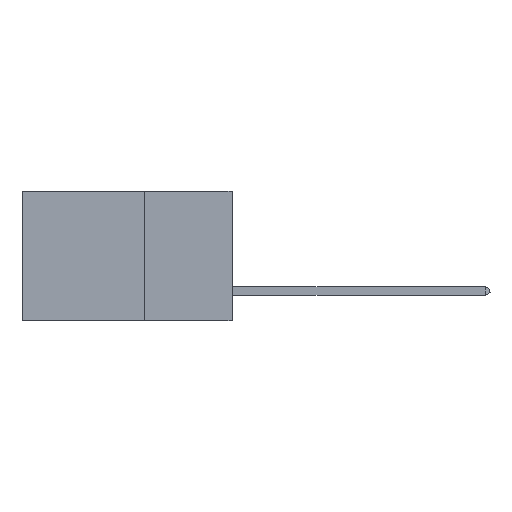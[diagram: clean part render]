
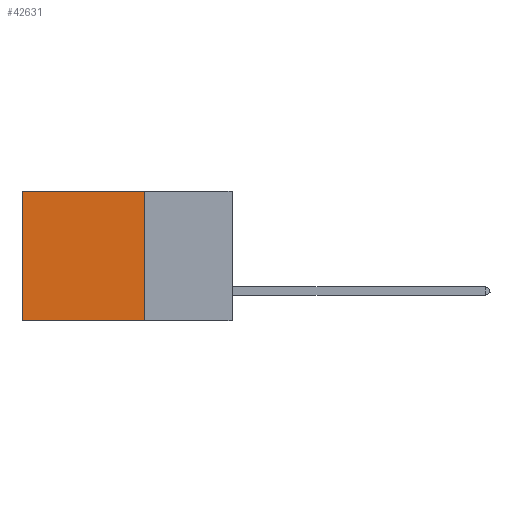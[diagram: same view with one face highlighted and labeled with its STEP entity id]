
A CAD part, left-side view. The second image highlights one B-rep face of the part: STEP entity #42631.
In plain terms, the highlighted planar face has unit normal (-1, 0, 0).
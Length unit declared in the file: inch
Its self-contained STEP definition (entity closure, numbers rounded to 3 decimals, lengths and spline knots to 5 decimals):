
#257 = EDGE_CURVE ( 'NONE', #31755, #35218, #38002, .T. ) ;
#869 = ORIENTED_EDGE ( 'NONE', *, *, #32308, .T. ) ;
#3611 = PLANE ( 'NONE',  #15359 ) ;
#4329 = DIRECTION ( 'NONE',  ( 0., 0., -1. ) ) ;
#5805 = EDGE_CURVE ( 'NONE', #31755, #28774, #27820, .T. ) ;
#6873 = VECTOR ( 'NONE', #4329, 39.37008 ) ;
#7428 = VECTOR ( 'NONE', #9564, 39.37008 ) ;
#7814 = CARTESIAN_POINT ( 'NONE',  ( 0.2875, 0.25, 0. ) ) ;
#9564 = DIRECTION ( 'NONE',  ( 0., 1., 0. ) ) ;
#13995 = DIRECTION ( 'NONE',  ( 1., 0., 0. ) ) ;
#14506 = CARTESIAN_POINT ( 'NONE',  ( 0.2875, 0.6, 0. ) ) ;
#14815 = VERTEX_POINT ( 'NONE', #32773 ) ;
#15359 = AXIS2_PLACEMENT_3D ( 'NONE', #34558, #13995, #31241 ) ;
#16577 = CARTESIAN_POINT ( 'NONE',  ( 0.2875, 0.25, 0. ) ) ;
#18350 = ORIENTED_EDGE ( 'NONE', *, *, #257, .F. ) ;
#19841 = ORIENTED_EDGE ( 'NONE', *, *, #38882, .F. ) ;
#22230 = CARTESIAN_POINT ( 'NONE',  ( 0.2875, 0.25, -0.37 ) ) ;
#23427 = CARTESIAN_POINT ( 'NONE',  ( 0.2875, 0.6, 0. ) ) ;
#23486 = CARTESIAN_POINT ( 'NONE',  ( 0.2875, 0.25, -0.37 ) ) ;
#25812 = FACE_OUTER_BOUND ( 'NONE', #38825, .T. ) ;
#27734 = LINE ( 'NONE', #23427, #30405 ) ;
#27820 = LINE ( 'NONE', #27873, #7428 ) ;
#27873 = CARTESIAN_POINT ( 'NONE',  ( 0.2875, 0.25, 0. ) ) ;
#28774 = VERTEX_POINT ( 'NONE', #14506 ) ;
#30405 = VECTOR ( 'NONE', #33788, 39.37008 ) ;
#31241 = DIRECTION ( 'NONE',  ( 0., 0., -1. ) ) ;
#31342 = VECTOR ( 'NONE', #37603, 39.37008 ) ;
#31755 = VERTEX_POINT ( 'NONE', #16577 ) ;
#32308 = EDGE_CURVE ( 'NONE', #28774, #14815, #27734, .T. ) ;
#32773 = CARTESIAN_POINT ( 'NONE',  ( 0.2875, 0.6, -0.37 ) ) ;
#33788 = DIRECTION ( 'NONE',  ( 0., 0., -1. ) ) ;
#34558 = CARTESIAN_POINT ( 'NONE',  ( 0.2875, 0.25, 0. ) ) ;
#34811 = ORIENTED_EDGE ( 'NONE', *, *, #5805, .T. ) ;
#35218 = VERTEX_POINT ( 'NONE', #22230 ) ;
#37603 = DIRECTION ( 'NONE',  ( 0., 1., 0. ) ) ;
#38002 = LINE ( 'NONE', #7814, #6873 ) ;
#38825 = EDGE_LOOP ( 'NONE', ( #869, #19841, #18350, #34811 ) ) ;
#38882 = EDGE_CURVE ( 'NONE', #35218, #14815, #40515, .T. ) ;
#40515 = LINE ( 'NONE', #23486, #31342 ) ;
#42631 = ADVANCED_FACE ( 'NONE', ( #25812 ), #3611, .F. ) ;
